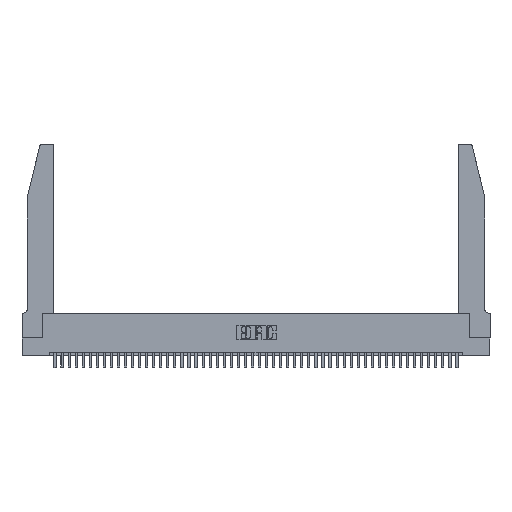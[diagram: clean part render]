
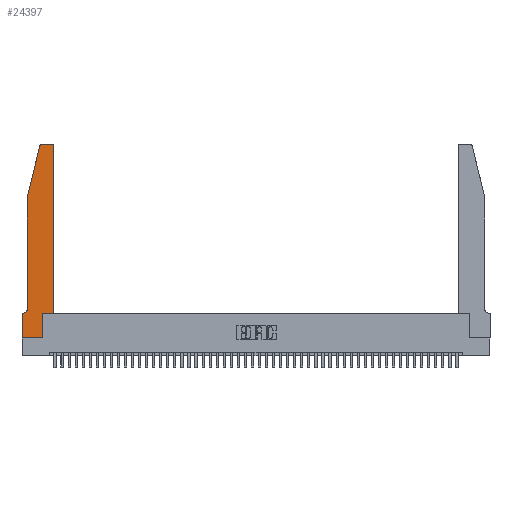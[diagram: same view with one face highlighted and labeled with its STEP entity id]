
A CAD part, top view. The second image highlights one B-rep face of the part: STEP entity #24397.
In plain terms, the highlighted planar face has unit normal (0, 0, 1).
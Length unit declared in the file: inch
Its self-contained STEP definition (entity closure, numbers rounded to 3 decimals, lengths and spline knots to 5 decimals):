
#80 = EDGE_CURVE ( 'NONE', #20179, #25289, #33920, .T. ) ;
#291 = CARTESIAN_POINT ( 'NONE',  ( 0., 0., 0.37 ) ) ;
#1658 = LINE ( 'NONE', #41641, #26146 ) ;
#1672 = VERTEX_POINT ( 'NONE', #3610 ) ;
#1873 = EDGE_CURVE ( 'NONE', #17613, #7461, #5126, .T. ) ;
#2175 = DIRECTION ( 'NONE',  ( 1., 0., 0. ) ) ;
#2627 = CARTESIAN_POINT ( 'NONE',  ( 0.4205, 2.75, 0.37 ) ) ;
#2718 = AXIS2_PLACEMENT_3D ( 'NONE', #42422, #20131, #5467 ) ;
#3073 = CIRCLE ( 'NONE', #47587, 0.07 ) ;
#3172 = DIRECTION ( 'NONE',  ( 0., 1., 0. ) ) ;
#3286 = DIRECTION ( 'NONE',  ( -1., 0., 0. ) ) ;
#3610 = CARTESIAN_POINT ( 'NONE',  ( 0.4505, 0.35, 0.37 ) ) ;
#4359 = DIRECTION ( 'NONE',  ( -0.239, -0.971, 0. ) ) ;
#4894 = VECTOR ( 'NONE', #3172, 39.37008 ) ;
#5083 = CARTESIAN_POINT ( 'NONE',  ( 0.4505, 2.72, 0.37 ) ) ;
#5126 = LINE ( 'NONE', #291, #23773 ) ;
#5428 = LINE ( 'NONE', #11968, #34032 ) ;
#5467 = DIRECTION ( 'NONE',  ( 1., 0., 0. ) ) ;
#5889 = VERTEX_POINT ( 'NONE', #35300 ) ;
#5998 = FACE_OUTER_BOUND ( 'NONE', #31644, .T. ) ;
#6145 = EDGE_CURVE ( 'NONE', #40641, #40839, #9793, .T. ) ;
#6866 = CARTESIAN_POINT ( 'NONE',  ( 0., 0.35, 0.37 ) ) ;
#7461 = VERTEX_POINT ( 'NONE', #12452 ) ;
#8161 = VERTEX_POINT ( 'NONE', #44422 ) ;
#8294 = EDGE_CURVE ( 'NONE', #8525, #8161, #12459, .T. ) ;
#8525 = VERTEX_POINT ( 'NONE', #39514 ) ;
#9101 = EDGE_CURVE ( 'NONE', #5889, #28982, #34620, .T. ) ;
#9415 = EDGE_CURVE ( 'NONE', #8161, #20179, #3073, .T. ) ;
#9793 = CIRCLE ( 'NONE', #31718, 0.03 ) ;
#10574 = ORIENTED_EDGE ( 'NONE', *, *, #6145, .T. ) ;
#11659 = EDGE_CURVE ( 'NONE', #25289, #17613, #24483, .T. ) ;
#11968 = CARTESIAN_POINT ( 'NONE',  ( 0.0755, 2., 0.37 ) ) ;
#12452 = CARTESIAN_POINT ( 'NONE',  ( 0.2865, 0., 0.37 ) ) ;
#12459 = LINE ( 'NONE', #41971, #35266 ) ;
#12774 = VERTEX_POINT ( 'NONE', #24714 ) ;
#12871 = ORIENTED_EDGE ( 'NONE', *, *, #9101, .T. ) ;
#15239 = DIRECTION ( 'NONE',  ( 1., 0., 0. ) ) ;
#15420 = DIRECTION ( 'NONE',  ( 0., -1., 0. ) ) ;
#15943 = LINE ( 'NONE', #44173, #4894 ) ;
#16800 = CARTESIAN_POINT ( 'NONE',  ( 0.284, 2.72, 0.37 ) ) ;
#17007 = ORIENTED_EDGE ( 'NONE', *, *, #38263, .T. ) ;
#17613 = VERTEX_POINT ( 'NONE', #25755 ) ;
#17763 = CARTESIAN_POINT ( 'NONE',  ( 0.2605, 2.75, 0.37 ) ) ;
#18412 = EDGE_CURVE ( 'NONE', #12774, #1672, #1658, .T. ) ;
#18587 = ORIENTED_EDGE ( 'NONE', *, *, #26350, .T. ) ;
#18857 = DIRECTION ( 'NONE',  ( 1., 0., 0. ) ) ;
#19297 = VECTOR ( 'NONE', #31777, 39.37008 ) ;
#19910 = ORIENTED_EDGE ( 'NONE', *, *, #1873, .T. ) ;
#20069 = CARTESIAN_POINT ( 'NONE',  ( 0.0055, 0.42, 0.37 ) ) ;
#20131 = DIRECTION ( 'NONE',  ( 0., 0., 1. ) ) ;
#20179 = VERTEX_POINT ( 'NONE', #29432 ) ;
#20278 = DIRECTION ( 'NONE',  ( 0., 1., 0. ) ) ;
#20957 = VECTOR ( 'NONE', #32822, 39.37008 ) ;
#23466 = ORIENTED_EDGE ( 'NONE', *, *, #9415, .T. ) ;
#23561 = ORIENTED_EDGE ( 'NONE', *, *, #24729, .T. ) ;
#23636 = CARTESIAN_POINT ( 'NONE',  ( 0.0755, 0.35, 0.37 ) ) ;
#23655 = DIRECTION ( 'NONE',  ( 0., 0., -1. ) ) ;
#23773 = VECTOR ( 'NONE', #18857, 39.37008 ) ;
#24397 = ADVANCED_FACE ( 'NONE', ( #5998 ), #38710, .T. ) ;
#24482 = DIRECTION ( 'NONE',  ( 0., 0., 1. ) ) ;
#24483 = LINE ( 'NONE', #32659, #20957 ) ;
#24714 = CARTESIAN_POINT ( 'NONE',  ( 0.2865, 0.35, 0.37 ) ) ;
#24729 = EDGE_CURVE ( 'NONE', #7461, #12774, #15943, .T. ) ;
#25289 = VERTEX_POINT ( 'NONE', #6866 ) ;
#25755 = CARTESIAN_POINT ( 'NONE',  ( 0., 0., 0.37 ) ) ;
#26146 = VECTOR ( 'NONE', #15239, 39.37008 ) ;
#26350 = EDGE_CURVE ( 'NONE', #28982, #8525, #5428, .T. ) ;
#28982 = VERTEX_POINT ( 'NONE', #44096 ) ;
#29432 = CARTESIAN_POINT ( 'NONE',  ( 0.0055, 0.35, 0.37 ) ) ;
#30925 = ORIENTED_EDGE ( 'NONE', *, *, #18412, .T. ) ;
#30999 = DIRECTION ( 'NONE',  ( -1., 0., 0. ) ) ;
#31603 = ORIENTED_EDGE ( 'NONE', *, *, #80, .T. ) ;
#31644 = EDGE_LOOP ( 'NONE', ( #45041, #12871, #18587, #40603, #23466, #31603, #42863, #19910, #23561, #30925, #17007, #10574 ) ) ;
#31718 = AXIS2_PLACEMENT_3D ( 'NONE', #34170, #34636, #38363 ) ;
#31777 = DIRECTION ( 'NONE',  ( -1., 0., 0. ) ) ;
#32659 = CARTESIAN_POINT ( 'NONE',  ( 0., 0., 0.37 ) ) ;
#32822 = DIRECTION ( 'NONE',  ( 0., -1., 0. ) ) ;
#33860 = LINE ( 'NONE', #42260, #37907 ) ;
#33920 = LINE ( 'NONE', #23636, #19297 ) ;
#34032 = VECTOR ( 'NONE', #4359, 39.37008 ) ;
#34170 = CARTESIAN_POINT ( 'NONE',  ( 0.4205, 2.72, 0.37 ) ) ;
#34620 = CIRCLE ( 'NONE', #40649, 0.03 ) ;
#34636 = DIRECTION ( 'NONE',  ( 0., 0., 1. ) ) ;
#35266 = VECTOR ( 'NONE', #15420, 39.37008 ) ;
#35300 = CARTESIAN_POINT ( 'NONE',  ( 0.284, 2.75, 0.37 ) ) ;
#35677 = LINE ( 'NONE', #17763, #40860 ) ;
#36730 = EDGE_CURVE ( 'NONE', #40839, #5889, #35677, .T. ) ;
#37907 = VECTOR ( 'NONE', #20278, 39.37008 ) ;
#38263 = EDGE_CURVE ( 'NONE', #1672, #40641, #33860, .T. ) ;
#38363 = DIRECTION ( 'NONE',  ( 1., 0., 0. ) ) ;
#38710 = PLANE ( 'NONE',  #2718 ) ;
#39514 = CARTESIAN_POINT ( 'NONE',  ( 0.0755, 2., 0.37 ) ) ;
#40603 = ORIENTED_EDGE ( 'NONE', *, *, #8294, .T. ) ;
#40641 = VERTEX_POINT ( 'NONE', #5083 ) ;
#40649 = AXIS2_PLACEMENT_3D ( 'NONE', #16800, #24482, #2175 ) ;
#40839 = VERTEX_POINT ( 'NONE', #2627 ) ;
#40860 = VECTOR ( 'NONE', #3286, 39.37008 ) ;
#41641 = CARTESIAN_POINT ( 'NONE',  ( 0.4505, 0.35, 0.37 ) ) ;
#41971 = CARTESIAN_POINT ( 'NONE',  ( 0.0755, 2., 0.37 ) ) ;
#42260 = CARTESIAN_POINT ( 'NONE',  ( 0.4505, 0.35, 0.37 ) ) ;
#42422 = CARTESIAN_POINT ( 'NONE',  ( 0., 0.35, 0.37 ) ) ;
#42863 = ORIENTED_EDGE ( 'NONE', *, *, #11659, .T. ) ;
#44096 = CARTESIAN_POINT ( 'NONE',  ( 0.25487, 2.72718, 0.37 ) ) ;
#44173 = CARTESIAN_POINT ( 'NONE',  ( 0.2865, 0.35, 0.37 ) ) ;
#44422 = CARTESIAN_POINT ( 'NONE',  ( 0.0755, 0.42, 0.37 ) ) ;
#45041 = ORIENTED_EDGE ( 'NONE', *, *, #36730, .T. ) ;
#47587 = AXIS2_PLACEMENT_3D ( 'NONE', #20069, #23655, #30999 ) ;
